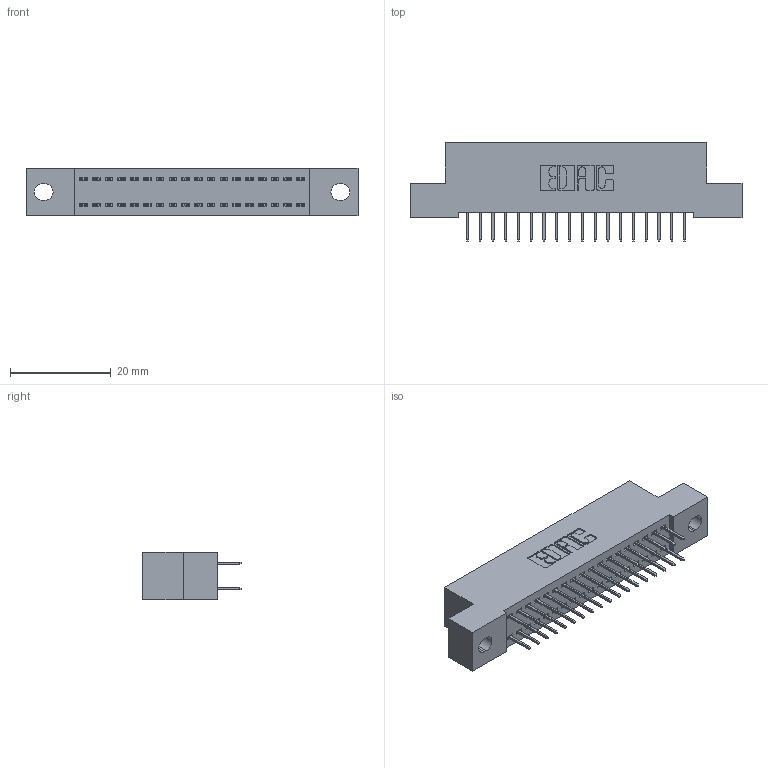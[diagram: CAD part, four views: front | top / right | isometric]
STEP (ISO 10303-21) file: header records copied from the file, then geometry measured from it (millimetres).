
FILE_DESCRIPTION (( 'STEP AP203' ), '1' );
FILE_NAME ('392-036-524-202.STEP', '2018-08-16T03:15:14', ( '' ), ( '' ), 'SwSTEP 2.0', 'SolidWorks 2016', '' );
FILE_SCHEMA (( 'CONFIG_CONTROL_DESIGN' ));
Length unit declared in the file: inch
Products named in the file (3): 342 Part_.128 Slot; 345-292-001_345-293-124; 392-036-524-202
Assembly tree (37 placements, depth 2):
  392-036-524-202
    342 Part_.128 Slot
    345-292-001_345-293-124  x36
Bounding box: 66.04 x 19.69 x 9.4 mm (x, y, z)
Volume: 5713.5 mm3; surface area: 8326.5 mm2
Topology: 37 solids, 37 shells, 2130 faces, 6035 edges, 3878 vertices
Faces by surface type: plane 1582, cylinder 548
Entity records: 14761 total; most frequent: CARTESIAN_POINT 2474, ORIENTED_EDGE 2410, DIRECTION 2157, EDGE_CURVE 1205, LINE 1081, VECTOR 1081, VERTEX_POINT 798, AXIS2_PLACEMENT_3D 538
